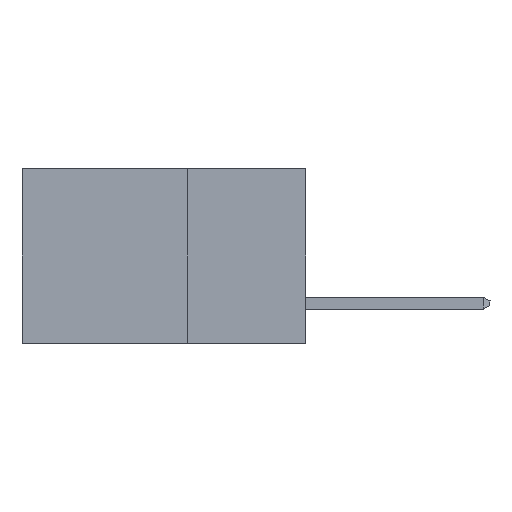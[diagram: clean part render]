
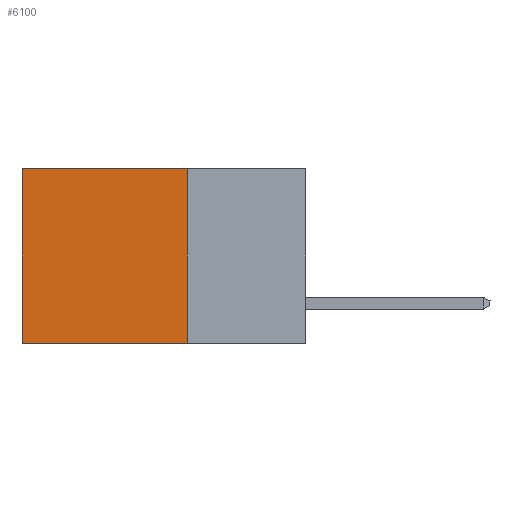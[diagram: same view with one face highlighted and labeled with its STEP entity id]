
A CAD part, left-side view. The second image highlights one B-rep face of the part: STEP entity #6100.
In plain terms, the highlighted planar face has unit normal (-1, 0, 0).
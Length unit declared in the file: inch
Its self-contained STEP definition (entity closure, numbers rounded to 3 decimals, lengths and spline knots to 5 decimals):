
#793 = VERTEX_POINT ( 'NONE', #4325 ) ;
#835 = VERTEX_POINT ( 'NONE', #9421 ) ;
#1004 = EDGE_CURVE ( 'NONE', #835, #793, #7186, .T. ) ;
#1946 = ORIENTED_EDGE ( 'NONE', *, *, #7687, .F. ) ;
#2133 = EDGE_CURVE ( 'NONE', #5887, #793, #8428, .T. ) ;
#3425 = AXIS2_PLACEMENT_3D ( 'NONE', #6253, #6168, #13432 ) ;
#3471 = CARTESIAN_POINT ( 'NONE',  ( 0.298, 0.25, 0. ) ) ;
#3792 = FACE_OUTER_BOUND ( 'NONE', #4891, .T. ) ;
#3924 = ORIENTED_EDGE ( 'NONE', *, *, #1004, .T. ) ;
#4321 = DIRECTION ( 'NONE',  ( 0., 0., -1. ) ) ;
#4325 = CARTESIAN_POINT ( 'NONE',  ( 0.298, 0.6, -0.37 ) ) ;
#4891 = EDGE_LOOP ( 'NONE', ( #3924, #11655, #1946, #7064 ) ) ;
#5887 = VERTEX_POINT ( 'NONE', #9145 ) ;
#6100 = ADVANCED_FACE ( 'NONE', ( #3792 ), #13270, .F. ) ;
#6168 = DIRECTION ( 'NONE',  ( 1., 0., 0. ) ) ;
#6253 = CARTESIAN_POINT ( 'NONE',  ( 0.298, 0.25, 0. ) ) ;
#7064 = ORIENTED_EDGE ( 'NONE', *, *, #7183, .T. ) ;
#7183 = EDGE_CURVE ( 'NONE', #12359, #835, #9250, .T. ) ;
#7186 = LINE ( 'NONE', #9242, #7985 ) ;
#7303 = VECTOR ( 'NONE', #9691, 39.37008 ) ;
#7687 = EDGE_CURVE ( 'NONE', #12359, #5887, #12863, .T. ) ;
#7893 = DIRECTION ( 'NONE',  ( 0., 1., 0. ) ) ;
#7985 = VECTOR ( 'NONE', #4321, 39.37008 ) ;
#8030 = CARTESIAN_POINT ( 'NONE',  ( 0.298, 0.25, -0.37 ) ) ;
#8103 = VECTOR ( 'NONE', #7893, 39.37008 ) ;
#8428 = LINE ( 'NONE', #8030, #13351 ) ;
#9145 = CARTESIAN_POINT ( 'NONE',  ( 0.298, 0.25, -0.37 ) ) ;
#9242 = CARTESIAN_POINT ( 'NONE',  ( 0.298, 0.6, 0. ) ) ;
#9250 = LINE ( 'NONE', #10861, #8103 ) ;
#9421 = CARTESIAN_POINT ( 'NONE',  ( 0.298, 0.6, 0. ) ) ;
#9691 = DIRECTION ( 'NONE',  ( 0., 0., -1. ) ) ;
#10861 = CARTESIAN_POINT ( 'NONE',  ( 0.298, 0.25, 0. ) ) ;
#11655 = ORIENTED_EDGE ( 'NONE', *, *, #2133, .F. ) ;
#11684 = CARTESIAN_POINT ( 'NONE',  ( 0.298, 0.25, 0. ) ) ;
#12359 = VERTEX_POINT ( 'NONE', #3471 ) ;
#12507 = DIRECTION ( 'NONE',  ( 0., 1., 0. ) ) ;
#12863 = LINE ( 'NONE', #11684, #7303 ) ;
#13270 = PLANE ( 'NONE',  #3425 ) ;
#13351 = VECTOR ( 'NONE', #12507, 39.37008 ) ;
#13432 = DIRECTION ( 'NONE',  ( 0., 0., -1. ) ) ;
